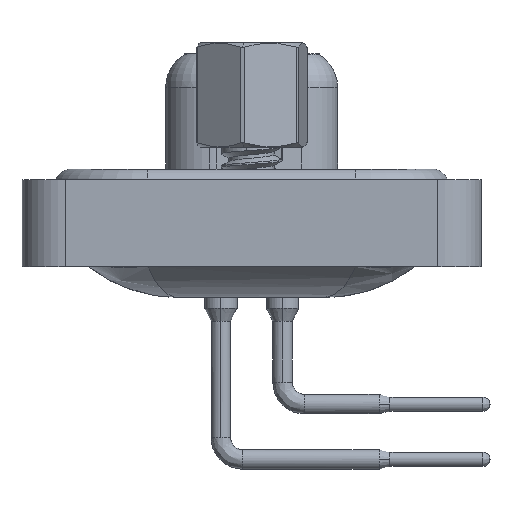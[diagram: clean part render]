
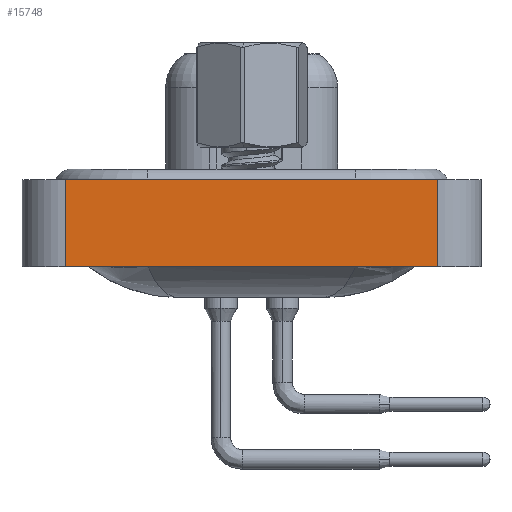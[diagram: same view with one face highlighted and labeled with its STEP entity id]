
A CAD part, left-side view. The second image highlights one B-rep face of the part: STEP entity #15748.
In plain terms, the highlighted planar face has unit normal (-1, 0, 0).
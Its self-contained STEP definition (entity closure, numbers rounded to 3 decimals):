
#34 = DIRECTION ( 'NONE',  ( 0., -1., 0. ) ) ;
#346 = VECTOR ( 'NONE', #3214, 1000. ) ;
#854 = CARTESIAN_POINT ( 'NONE',  ( -7.35, -8.55, -3.6 ) ) ;
#1339 = PLANE ( 'NONE',  #7920 ) ;
#1772 = CARTESIAN_POINT ( 'NONE',  ( -7.35, -8.55, 0.4 ) ) ;
#2345 = LINE ( 'NONE', #6733, #10842 ) ;
#2629 = EDGE_CURVE ( 'NONE', #17998, #9525, #2345, .T. ) ;
#3214 = DIRECTION ( 'NONE',  ( 0., 0., 1. ) ) ;
#3595 = VECTOR ( 'NONE', #34, 1000. ) ;
#6599 = CARTESIAN_POINT ( 'NONE',  ( -7.35, -8.55, -3.6 ) ) ;
#6733 = CARTESIAN_POINT ( 'NONE',  ( -7.35, -8.55, 0.4 ) ) ;
#7603 = DIRECTION ( 'NONE',  ( 0., 0., 1. ) ) ;
#7920 = AXIS2_PLACEMENT_3D ( 'NONE', #10269, #21617, #23688 ) ;
#8482 = ORIENTED_EDGE ( 'NONE', *, *, #18141, .T. ) ;
#8499 = DIRECTION ( 'NONE',  ( 0., -1., 0. ) ) ;
#9238 = EDGE_LOOP ( 'NONE', ( #25798, #10527, #13080, #8482 ) ) ;
#9525 = VERTEX_POINT ( 'NONE', #1772 ) ;
#10269 = CARTESIAN_POINT ( 'NONE',  ( -7.35, -8.55, -3.6 ) ) ;
#10527 = ORIENTED_EDGE ( 'NONE', *, *, #2629, .F. ) ;
#10842 = VECTOR ( 'NONE', #8499, 1000. ) ;
#11122 = VECTOR ( 'NONE', #7603, 1000. ) ;
#12637 = EDGE_CURVE ( 'NONE', #15334, #17998, #23365, .T. ) ;
#13080 = ORIENTED_EDGE ( 'NONE', *, *, #12637, .F. ) ;
#15334 = VERTEX_POINT ( 'NONE', #17426 ) ;
#15748 = ADVANCED_FACE ( 'NONE', ( #23828 ), #1339, .T. ) ;
#17008 = CARTESIAN_POINT ( 'NONE',  ( -7.35, 8.55, 0.4 ) ) ;
#17426 = CARTESIAN_POINT ( 'NONE',  ( -7.35, 8.55, -3.6 ) ) ;
#17998 = VERTEX_POINT ( 'NONE', #17008 ) ;
#18141 = EDGE_CURVE ( 'NONE', #15334, #18695, #19484, .T. ) ;
#18695 = VERTEX_POINT ( 'NONE', #6599 ) ;
#18984 = CARTESIAN_POINT ( 'NONE',  ( -7.35, 8.55, -3.6 ) ) ;
#19216 = EDGE_CURVE ( 'NONE', #18695, #9525, #21669, .T. ) ;
#19484 = LINE ( 'NONE', #21662, #3595 ) ;
#21617 = DIRECTION ( 'NONE',  ( -1., 0., 0. ) ) ;
#21662 = CARTESIAN_POINT ( 'NONE',  ( -7.35, -8.55, -3.6 ) ) ;
#21669 = LINE ( 'NONE', #854, #11122 ) ;
#23365 = LINE ( 'NONE', #18984, #346 ) ;
#23688 = DIRECTION ( 'NONE',  ( 0., 0., 1. ) ) ;
#23828 = FACE_OUTER_BOUND ( 'NONE', #9238, .T. ) ;
#25798 = ORIENTED_EDGE ( 'NONE', *, *, #19216, .T. ) ;
